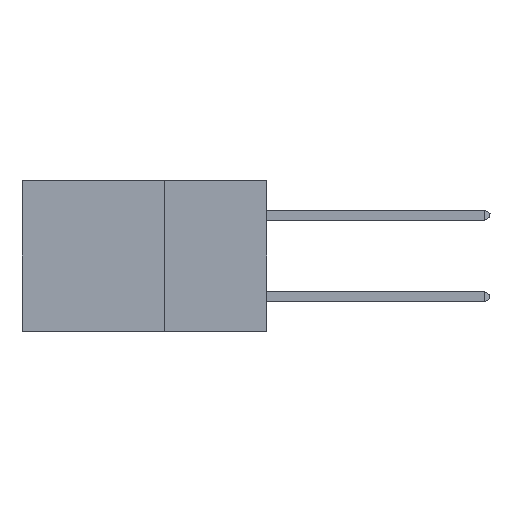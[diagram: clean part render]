
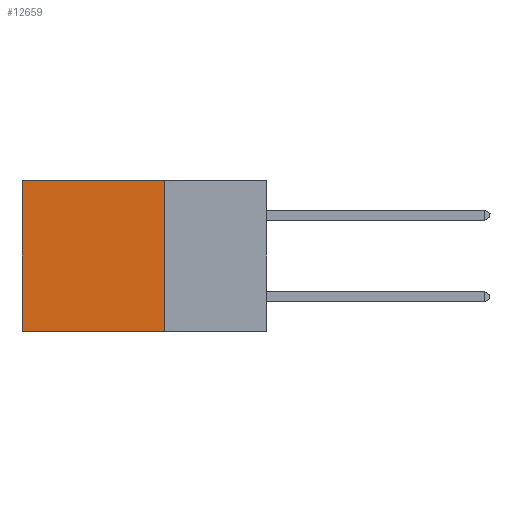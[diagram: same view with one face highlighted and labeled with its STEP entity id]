
A CAD part, left-side view. The second image highlights one B-rep face of the part: STEP entity #12659.
In plain terms, the highlighted planar face has unit normal (-1, 0, 0).
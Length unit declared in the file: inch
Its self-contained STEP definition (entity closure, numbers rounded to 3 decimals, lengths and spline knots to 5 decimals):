
#294 = DIRECTION ( 'NONE',  ( 0., 1., 0. ) ) ;
#1079 = ORIENTED_EDGE ( 'NONE', *, *, #11382, .T. ) ;
#1226 = CARTESIAN_POINT ( 'NONE',  ( 0.2875, 0.25, 0. ) ) ;
#1705 = ORIENTED_EDGE ( 'NONE', *, *, #26154, .F. ) ;
#2995 = ORIENTED_EDGE ( 'NONE', *, *, #18601, .F. ) ;
#5244 = EDGE_CURVE ( 'NONE', #25035, #27108, #20885, .T. ) ;
#6840 = DIRECTION ( 'NONE',  ( 0., 0., -1. ) ) ;
#8018 = CARTESIAN_POINT ( 'NONE',  ( 0.2875, 0.6, 0. ) ) ;
#8251 = FACE_OUTER_BOUND ( 'NONE', #19856, .T. ) ;
#9477 = LINE ( 'NONE', #18798, #27058 ) ;
#9954 = AXIS2_PLACEMENT_3D ( 'NONE', #1226, #12400, #21701 ) ;
#10525 = CARTESIAN_POINT ( 'NONE',  ( 0.2875, 0.6, 0. ) ) ;
#10988 = CARTESIAN_POINT ( 'NONE',  ( 0.2875, 0.25, 0. ) ) ;
#11361 = VERTEX_POINT ( 'NONE', #28995 ) ;
#11382 = EDGE_CURVE ( 'NONE', #27108, #29971, #12806, .T. ) ;
#11921 = CARTESIAN_POINT ( 'NONE',  ( 0.2875, 0.25, 0. ) ) ;
#12400 = DIRECTION ( 'NONE',  ( 1., 0., 0. ) ) ;
#12659 = ADVANCED_FACE ( 'NONE', ( #8251 ), #17117, .F. ) ;
#12806 = LINE ( 'NONE', #10525, #23540 ) ;
#14053 = CARTESIAN_POINT ( 'NONE',  ( 0.2875, 0.6, -0.37 ) ) ;
#17117 = PLANE ( 'NONE',  #9954 ) ;
#18324 = ORIENTED_EDGE ( 'NONE', *, *, #5244, .T. ) ;
#18601 = EDGE_CURVE ( 'NONE', #25035, #11361, #25347, .T. ) ;
#18798 = CARTESIAN_POINT ( 'NONE',  ( 0.2875, 0.25, -0.37 ) ) ;
#19152 = VECTOR ( 'NONE', #6840, 39.37008 ) ;
#19706 = VECTOR ( 'NONE', #28063, 39.37008 ) ;
#19836 = DIRECTION ( 'NONE',  ( 0., 0., -1. ) ) ;
#19856 = EDGE_LOOP ( 'NONE', ( #1079, #1705, #2995, #18324 ) ) ;
#20885 = LINE ( 'NONE', #25788, #19706 ) ;
#21701 = DIRECTION ( 'NONE',  ( 0., 0., -1. ) ) ;
#23540 = VECTOR ( 'NONE', #19836, 39.37008 ) ;
#25035 = VERTEX_POINT ( 'NONE', #10988 ) ;
#25347 = LINE ( 'NONE', #11921, #19152 ) ;
#25788 = CARTESIAN_POINT ( 'NONE',  ( 0.2875, 0.25, 0. ) ) ;
#26154 = EDGE_CURVE ( 'NONE', #11361, #29971, #9477, .T. ) ;
#27058 = VECTOR ( 'NONE', #294, 39.37008 ) ;
#27108 = VERTEX_POINT ( 'NONE', #8018 ) ;
#28063 = DIRECTION ( 'NONE',  ( 0., 1., 0. ) ) ;
#28995 = CARTESIAN_POINT ( 'NONE',  ( 0.2875, 0.25, -0.37 ) ) ;
#29971 = VERTEX_POINT ( 'NONE', #14053 ) ;
